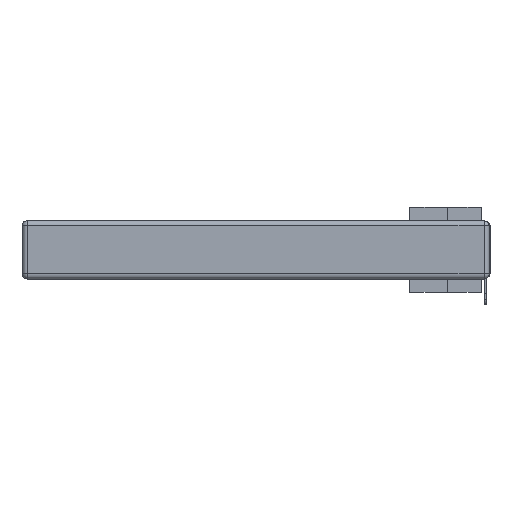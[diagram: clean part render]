
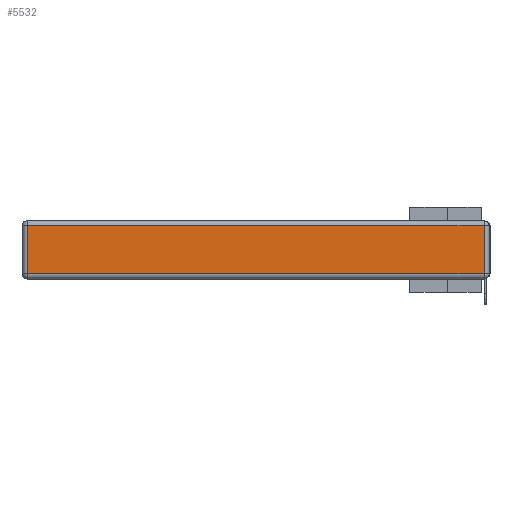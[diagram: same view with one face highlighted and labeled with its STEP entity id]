
A CAD part, left-side view. The second image highlights one B-rep face of the part: STEP entity #5532.
In plain terms, the highlighted planar face has unit normal (-1, 0, 0).
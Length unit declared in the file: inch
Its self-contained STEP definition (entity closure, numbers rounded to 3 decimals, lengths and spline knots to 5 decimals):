
#2346 = VERTEX_POINT ( 'NONE', #24583 ) ;
#2523 = CARTESIAN_POINT ( 'NONE',  ( 0., 0.03, -0.313 ) ) ;
#3025 = AXIS2_PLACEMENT_3D ( 'NONE', #21550, #26340, #19199 ) ;
#4112 = VECTOR ( 'NONE', #27577, 39.37008 ) ;
#5532 = ADVANCED_FACE ( 'NONE', ( #7322 ), #9267, .T. ) ;
#6895 = EDGE_CURVE ( 'NONE', #19209, #7059, #25319, .T. ) ;
#7059 = VERTEX_POINT ( 'NONE', #10104 ) ;
#7157 = DIRECTION ( 'NONE',  ( 0., 1., 0. ) ) ;
#7322 = FACE_OUTER_BOUND ( 'NONE', #16412, .T. ) ;
#9267 = PLANE ( 'NONE',  #3025 ) ;
#10104 = CARTESIAN_POINT ( 'NONE',  ( 0., 2.72, -0.313 ) ) ;
#10142 = VECTOR ( 'NONE', #17991, 39.37008 ) ;
#14537 = CARTESIAN_POINT ( 'NONE',  ( 0., 2.72, -0.343 ) ) ;
#15220 = CARTESIAN_POINT ( 'NONE',  ( 0., 0.03, -0.343 ) ) ;
#16412 = EDGE_LOOP ( 'NONE', ( #16437, #29405, #22632, #23346 ) ) ;
#16437 = ORIENTED_EDGE ( 'NONE', *, *, #17980, .T. ) ;
#16872 = CARTESIAN_POINT ( 'NONE',  ( 0., 2.75, -0.03 ) ) ;
#17235 = CARTESIAN_POINT ( 'NONE',  ( 0., 0., -0.313 ) ) ;
#17651 = EDGE_CURVE ( 'NONE', #31508, #2346, #26601, .T. ) ;
#17980 = EDGE_CURVE ( 'NONE', #7059, #31508, #27321, .T. ) ;
#17991 = DIRECTION ( 'NONE',  ( 0., -1., 0. ) ) ;
#18881 = VECTOR ( 'NONE', #24328, 39.37008 ) ;
#19199 = DIRECTION ( 'NONE',  ( 0., 0., 1. ) ) ;
#19209 = VERTEX_POINT ( 'NONE', #24229 ) ;
#20679 = VECTOR ( 'NONE', #7157, 39.37008 ) ;
#21469 = LINE ( 'NONE', #16872, #20679 ) ;
#21550 = CARTESIAN_POINT ( 'NONE',  ( 0., 0., -0.343 ) ) ;
#22632 = ORIENTED_EDGE ( 'NONE', *, *, #29060, .T. ) ;
#23346 = ORIENTED_EDGE ( 'NONE', *, *, #6895, .T. ) ;
#24229 = CARTESIAN_POINT ( 'NONE',  ( 0., 2.72, -0.03 ) ) ;
#24328 = DIRECTION ( 'NONE',  ( 0., 0., -1. ) ) ;
#24583 = CARTESIAN_POINT ( 'NONE',  ( 0., 0.03, -0.03 ) ) ;
#25319 = LINE ( 'NONE', #14537, #18881 ) ;
#26340 = DIRECTION ( 'NONE',  ( -1., 0., 0. ) ) ;
#26601 = LINE ( 'NONE', #15220, #4112 ) ;
#27321 = LINE ( 'NONE', #17235, #10142 ) ;
#27577 = DIRECTION ( 'NONE',  ( 0., 0., 1. ) ) ;
#29060 = EDGE_CURVE ( 'NONE', #2346, #19209, #21469, .T. ) ;
#29405 = ORIENTED_EDGE ( 'NONE', *, *, #17651, .T. ) ;
#31508 = VERTEX_POINT ( 'NONE', #2523 ) ;
